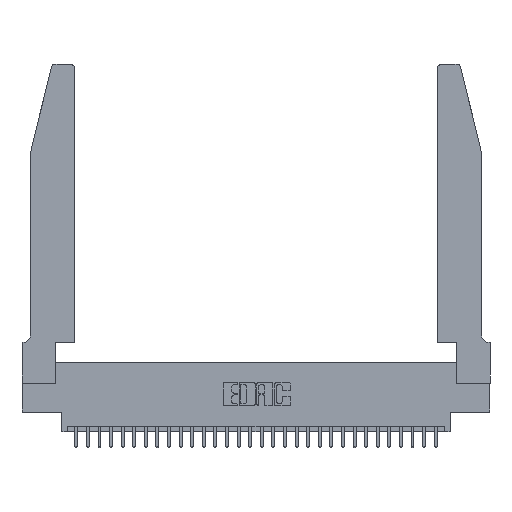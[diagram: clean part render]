
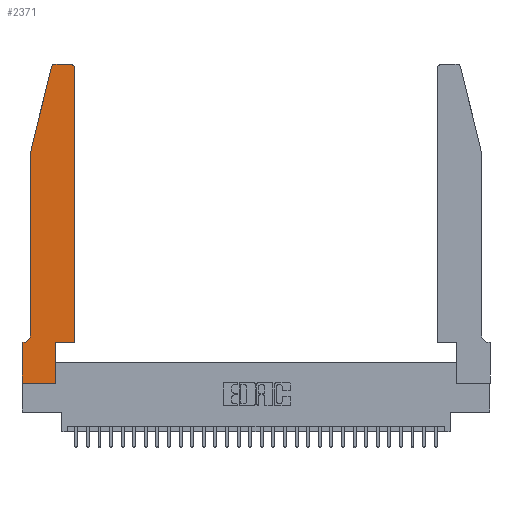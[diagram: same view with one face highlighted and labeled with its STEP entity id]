
A CAD part, top view. The second image highlights one B-rep face of the part: STEP entity #2371.
In plain terms, the highlighted planar face has unit normal (0, 0, 1).
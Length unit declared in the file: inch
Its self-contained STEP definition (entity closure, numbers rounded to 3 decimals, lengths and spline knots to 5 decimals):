
#128 = VERTEX_POINT ( 'NONE', #17922 ) ;
#480 = VECTOR ( 'NONE', #9334, 39.37008 ) ;
#931 = CARTESIAN_POINT ( 'NONE',  ( 0.4205, 2.72, 0.37 ) ) ;
#995 = ORIENTED_EDGE ( 'NONE', *, *, #3150, .T. ) ;
#1100 = CARTESIAN_POINT ( 'NONE',  ( 0.4505, 0.35, 0.37 ) ) ;
#1130 = LINE ( 'NONE', #6085, #19147 ) ;
#1150 = CARTESIAN_POINT ( 'NONE',  ( 0.25487, 2.72718, 0.37 ) ) ;
#1407 = DIRECTION ( 'NONE',  ( 0., -1., 0. ) ) ;
#1446 = VECTOR ( 'NONE', #8243, 39.37008 ) ;
#2070 = CARTESIAN_POINT ( 'NONE',  ( 0.0755, 2., 0.37 ) ) ;
#2195 = LINE ( 'NONE', #13218, #1446 ) ;
#2371 = ADVANCED_FACE ( 'NONE', ( #28231 ), #8058, .T. ) ;
#2439 = CARTESIAN_POINT ( 'NONE',  ( 0.4505, 2.72, 0.37 ) ) ;
#3000 = ORIENTED_EDGE ( 'NONE', *, *, #15716, .T. ) ;
#3150 = EDGE_CURVE ( 'NONE', #28583, #8054, #15035, .T. ) ;
#3356 = VERTEX_POINT ( 'NONE', #14369 ) ;
#3367 = DIRECTION ( 'NONE',  ( 1., 0., 0. ) ) ;
#3432 = VERTEX_POINT ( 'NONE', #2439 ) ;
#3844 = CARTESIAN_POINT ( 'NONE',  ( 0.0755, 2., 0.37 ) ) ;
#4388 = LINE ( 'NONE', #11796, #21601 ) ;
#4675 = VERTEX_POINT ( 'NONE', #8903 ) ;
#5425 = LINE ( 'NONE', #21494, #480 ) ;
#5435 = DIRECTION ( 'NONE',  ( -1., 0., 0. ) ) ;
#5822 = VERTEX_POINT ( 'NONE', #13255 ) ;
#6085 = CARTESIAN_POINT ( 'NONE',  ( 0.2865, 0.35, 0.37 ) ) ;
#7842 = ORIENTED_EDGE ( 'NONE', *, *, #9885, .T. ) ;
#8023 = EDGE_CURVE ( 'NONE', #12742, #28583, #5425, .T. ) ;
#8054 = VERTEX_POINT ( 'NONE', #23958 ) ;
#8058 = PLANE ( 'NONE',  #27100 ) ;
#8243 = DIRECTION ( 'NONE',  ( 1., 0., 0. ) ) ;
#8529 = ORIENTED_EDGE ( 'NONE', *, *, #15709, .T. ) ;
#8725 = VECTOR ( 'NONE', #18245, 39.37008 ) ;
#8903 = CARTESIAN_POINT ( 'NONE',  ( 0.0055, 0.35, 0.37 ) ) ;
#9058 = CARTESIAN_POINT ( 'NONE',  ( 0.284, 2.72, 0.37 ) ) ;
#9321 = ORIENTED_EDGE ( 'NONE', *, *, #19362, .T. ) ;
#9334 = DIRECTION ( 'NONE',  ( -0.239, -0.971, 0. ) ) ;
#9885 = EDGE_CURVE ( 'NONE', #15006, #10193, #1130, .T. ) ;
#9893 = CARTESIAN_POINT ( 'NONE',  ( 0.0755, 0.35, 0.37 ) ) ;
#10193 = VERTEX_POINT ( 'NONE', #25626 ) ;
#10777 = ORIENTED_EDGE ( 'NONE', *, *, #27072, .T. ) ;
#11129 = LINE ( 'NONE', #9893, #28849 ) ;
#11541 = DIRECTION ( 'NONE',  ( 1., 0., 0. ) ) ;
#11796 = CARTESIAN_POINT ( 'NONE',  ( 0., 0., 0.37 ) ) ;
#12394 = DIRECTION ( 'NONE',  ( -1., 0., 0. ) ) ;
#12742 = VERTEX_POINT ( 'NONE', #1150 ) ;
#13043 = DIRECTION ( 'NONE',  ( 0., 0., 1. ) ) ;
#13218 = CARTESIAN_POINT ( 'NONE',  ( 0.4505, 0.35, 0.37 ) ) ;
#13255 = CARTESIAN_POINT ( 'NONE',  ( 0.4505, 0.35, 0.37 ) ) ;
#13400 = EDGE_CURVE ( 'NONE', #29940, #12742, #15104, .T. ) ;
#14246 = DIRECTION ( 'NONE',  ( 0., -1., 0. ) ) ;
#14369 = CARTESIAN_POINT ( 'NONE',  ( 0., 0.35, 0.37 ) ) ;
#14494 = LINE ( 'NONE', #1100, #8725 ) ;
#14522 = CARTESIAN_POINT ( 'NONE',  ( 0.0055, 0.42, 0.37 ) ) ;
#14685 = VECTOR ( 'NONE', #21603, 39.37008 ) ;
#15006 = VERTEX_POINT ( 'NONE', #20691 ) ;
#15035 = LINE ( 'NONE', #3844, #21487 ) ;
#15104 = CIRCLE ( 'NONE', #28287, 0.03 ) ;
#15397 = VECTOR ( 'NONE', #5435, 39.37008 ) ;
#15709 = EDGE_CURVE ( 'NONE', #10193, #5822, #2195, .T. ) ;
#15716 = EDGE_CURVE ( 'NONE', #5822, #3432, #14494, .T. ) ;
#16200 = VERTEX_POINT ( 'NONE', #27886 ) ;
#16473 = ORIENTED_EDGE ( 'NONE', *, *, #29905, .T. ) ;
#16750 = CARTESIAN_POINT ( 'NONE',  ( 0., 0., 0.37 ) ) ;
#16995 = DIRECTION ( 'NONE',  ( -1., 0., 0. ) ) ;
#17704 = CARTESIAN_POINT ( 'NONE',  ( 0.2605, 2.75, 0.37 ) ) ;
#17922 = CARTESIAN_POINT ( 'NONE',  ( 0.4205, 2.75, 0.37 ) ) ;
#18006 = EDGE_CURVE ( 'NONE', #3432, #128, #29048, .T. ) ;
#18078 = DIRECTION ( 'NONE',  ( 0., 0., 1. ) ) ;
#18245 = DIRECTION ( 'NONE',  ( 0., 1., 0. ) ) ;
#18354 = EDGE_CURVE ( 'NONE', #8054, #4675, #30518, .T. ) ;
#19147 = VECTOR ( 'NONE', #20745, 39.37008 ) ;
#19362 = EDGE_CURVE ( 'NONE', #16200, #15006, #27466, .T. ) ;
#19962 = AXIS2_PLACEMENT_3D ( 'NONE', #14522, #31298, #16995 ) ;
#20564 = AXIS2_PLACEMENT_3D ( 'NONE', #931, #18078, #3367 ) ;
#20691 = CARTESIAN_POINT ( 'NONE',  ( 0.2865, 0., 0.37 ) ) ;
#20745 = DIRECTION ( 'NONE',  ( 0., 1., 0. ) ) ;
#21311 = ORIENTED_EDGE ( 'NONE', *, *, #8023, .T. ) ;
#21402 = ORIENTED_EDGE ( 'NONE', *, *, #13400, .T. ) ;
#21429 = EDGE_LOOP ( 'NONE', ( #25934, #21402, #21311, #995, #23060, #10777, #16473, #9321, #7842, #8529, #3000, #29228 ) ) ;
#21487 = VECTOR ( 'NONE', #1407, 39.37008 ) ;
#21494 = CARTESIAN_POINT ( 'NONE',  ( 0.0755, 2., 0.37 ) ) ;
#21601 = VECTOR ( 'NONE', #14246, 39.37008 ) ;
#21603 = DIRECTION ( 'NONE',  ( 1., 0., 0. ) ) ;
#22114 = EDGE_CURVE ( 'NONE', #128, #29940, #28900, .T. ) ;
#23060 = ORIENTED_EDGE ( 'NONE', *, *, #18354, .T. ) ;
#23958 = CARTESIAN_POINT ( 'NONE',  ( 0.0755, 0.42, 0.37 ) ) ;
#25626 = CARTESIAN_POINT ( 'NONE',  ( 0.2865, 0.35, 0.37 ) ) ;
#25934 = ORIENTED_EDGE ( 'NONE', *, *, #22114, .T. ) ;
#26003 = DIRECTION ( 'NONE',  ( 0., 0., 1. ) ) ;
#27072 = EDGE_CURVE ( 'NONE', #4675, #3356, #11129, .T. ) ;
#27100 = AXIS2_PLACEMENT_3D ( 'NONE', #27462, #13043, #29845 ) ;
#27462 = CARTESIAN_POINT ( 'NONE',  ( 0., 0.35, 0.37 ) ) ;
#27466 = LINE ( 'NONE', #16750, #14685 ) ;
#27886 = CARTESIAN_POINT ( 'NONE',  ( 0., 0., 0.37 ) ) ;
#28231 = FACE_OUTER_BOUND ( 'NONE', #21429, .T. ) ;
#28287 = AXIS2_PLACEMENT_3D ( 'NONE', #9058, #26003, #11541 ) ;
#28583 = VERTEX_POINT ( 'NONE', #2070 ) ;
#28849 = VECTOR ( 'NONE', #12394, 39.37008 ) ;
#28900 = LINE ( 'NONE', #17704, #15397 ) ;
#29048 = CIRCLE ( 'NONE', #20564, 0.03 ) ;
#29228 = ORIENTED_EDGE ( 'NONE', *, *, #18006, .T. ) ;
#29845 = DIRECTION ( 'NONE',  ( 1., 0., 0. ) ) ;
#29905 = EDGE_CURVE ( 'NONE', #3356, #16200, #4388, .T. ) ;
#29940 = VERTEX_POINT ( 'NONE', #31131 ) ;
#30518 = CIRCLE ( 'NONE', #19962, 0.07 ) ;
#31131 = CARTESIAN_POINT ( 'NONE',  ( 0.284, 2.75, 0.37 ) ) ;
#31298 = DIRECTION ( 'NONE',  ( 0., 0., -1. ) ) ;
